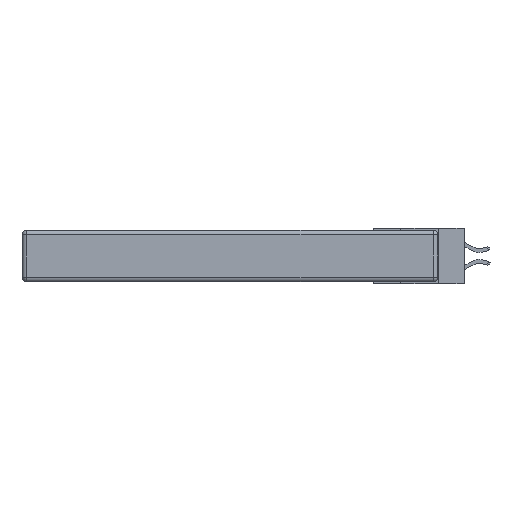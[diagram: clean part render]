
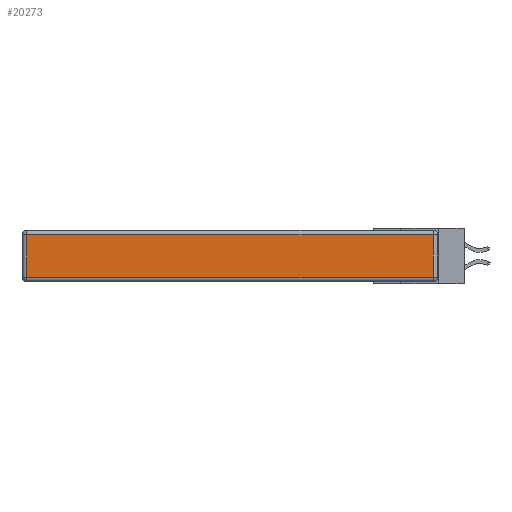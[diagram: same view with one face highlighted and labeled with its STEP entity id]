
A CAD part, left-side view. The second image highlights one B-rep face of the part: STEP entity #20273.
In plain terms, the highlighted planar face has unit normal (-1, 0, 0).
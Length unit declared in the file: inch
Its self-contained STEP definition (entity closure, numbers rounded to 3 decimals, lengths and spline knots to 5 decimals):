
#942 = CARTESIAN_POINT ( 'NONE',  ( 0., 2.72, -0.343 ) ) ;
#1365 = VECTOR ( 'NONE', #15600, 39.37008 ) ;
#3535 = VERTEX_POINT ( 'NONE', #6640 ) ;
#3808 = EDGE_CURVE ( 'NONE', #8210, #19897, #17951, .T. ) ;
#3857 = CARTESIAN_POINT ( 'NONE',  ( 0., 2.72, -0.03 ) ) ;
#5167 = ORIENTED_EDGE ( 'NONE', *, *, #12691, .T. ) ;
#5346 = LINE ( 'NONE', #9553, #1365 ) ;
#6640 = CARTESIAN_POINT ( 'NONE',  ( 0., 2.72, -0.313 ) ) ;
#6673 = LINE ( 'NONE', #16515, #10367 ) ;
#7087 = CARTESIAN_POINT ( 'NONE',  ( 0., 0.03, -0.03 ) ) ;
#7493 = DIRECTION ( 'NONE',  ( 0., 1., 0. ) ) ;
#8210 = VERTEX_POINT ( 'NONE', #7087 ) ;
#8557 = DIRECTION ( 'NONE',  ( -1., 0., 0. ) ) ;
#8839 = VECTOR ( 'NONE', #14639, 39.37008 ) ;
#9553 = CARTESIAN_POINT ( 'NONE',  ( 0., 0., -0.313 ) ) ;
#10367 = VECTOR ( 'NONE', #22452, 39.37008 ) ;
#11315 = LINE ( 'NONE', #942, #8839 ) ;
#11914 = CARTESIAN_POINT ( 'NONE',  ( 0., 0., -0.343 ) ) ;
#12691 = EDGE_CURVE ( 'NONE', #18215, #8210, #6673, .T. ) ;
#12765 = VECTOR ( 'NONE', #7493, 39.37008 ) ;
#13868 = DIRECTION ( 'NONE',  ( 0., 0., 1. ) ) ;
#14639 = DIRECTION ( 'NONE',  ( 0., 0., -1. ) ) ;
#15600 = DIRECTION ( 'NONE',  ( 0., -1., 0. ) ) ;
#16515 = CARTESIAN_POINT ( 'NONE',  ( 0., 0.03, -0.343 ) ) ;
#17769 = ORIENTED_EDGE ( 'NONE', *, *, #22721, .T. ) ;
#17780 = CARTESIAN_POINT ( 'NONE',  ( 0., 0.03, -0.313 ) ) ;
#17951 = LINE ( 'NONE', #24954, #12765 ) ;
#18215 = VERTEX_POINT ( 'NONE', #17780 ) ;
#18447 = EDGE_CURVE ( 'NONE', #19897, #3535, #11315, .T. ) ;
#18800 = ORIENTED_EDGE ( 'NONE', *, *, #18447, .T. ) ;
#18823 = FACE_OUTER_BOUND ( 'NONE', #18841, .T. ) ;
#18841 = EDGE_LOOP ( 'NONE', ( #17769, #5167, #20654, #18800 ) ) ;
#19897 = VERTEX_POINT ( 'NONE', #3857 ) ;
#20273 = ADVANCED_FACE ( 'NONE', ( #18823 ), #21576, .T. ) ;
#20654 = ORIENTED_EDGE ( 'NONE', *, *, #3808, .T. ) ;
#21576 = PLANE ( 'NONE',  #22252 ) ;
#22252 = AXIS2_PLACEMENT_3D ( 'NONE', #11914, #8557, #13868 ) ;
#22452 = DIRECTION ( 'NONE',  ( 0., 0., 1. ) ) ;
#22721 = EDGE_CURVE ( 'NONE', #3535, #18215, #5346, .T. ) ;
#24954 = CARTESIAN_POINT ( 'NONE',  ( 0., 2.75, -0.03 ) ) ;
